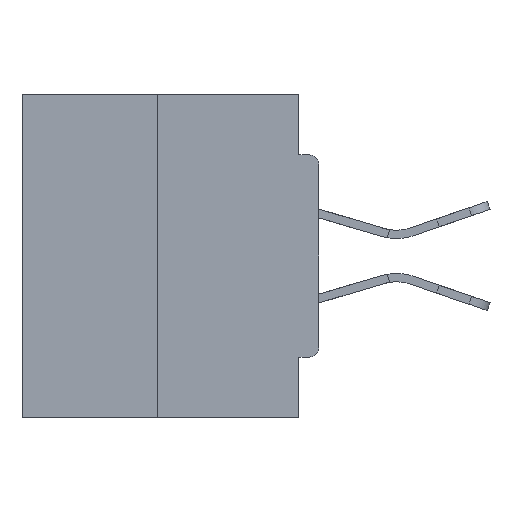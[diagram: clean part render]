
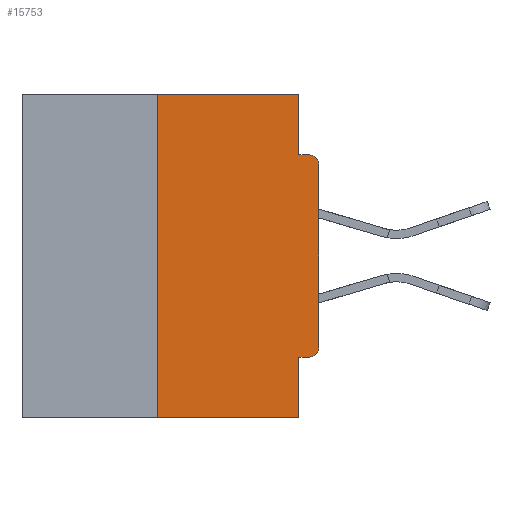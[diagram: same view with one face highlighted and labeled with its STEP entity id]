
A CAD part, left-side view. The second image highlights one B-rep face of the part: STEP entity #15753.
In plain terms, the highlighted planar face has unit normal (-1, 0, 0).
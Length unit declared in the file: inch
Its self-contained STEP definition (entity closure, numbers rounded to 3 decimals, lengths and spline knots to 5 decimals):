
#623 = VECTOR ( 'NONE', #2647, 39.37008 ) ;
#1178 = DIRECTION ( 'NONE',  ( 0., 0., -1. ) ) ;
#2207 = DIRECTION ( 'NONE',  ( 0., -1., 0. ) ) ;
#2476 = VERTEX_POINT ( 'NONE', #34500 ) ;
#2647 = DIRECTION ( 'NONE',  ( 0., 0., 1. ) ) ;
#2746 = VERTEX_POINT ( 'NONE', #12553 ) ;
#2925 = ORIENTED_EDGE ( 'NONE', *, *, #17171, .F. ) ;
#4962 = ORIENTED_EDGE ( 'NONE', *, *, #29750, .T. ) ;
#5063 = CARTESIAN_POINT ( 'NONE',  ( 0., 0., -0.3915 ) ) ;
#5082 = ORIENTED_EDGE ( 'NONE', *, *, #13976, .F. ) ;
#6606 = VERTEX_POINT ( 'NONE', #25374 ) ;
#6921 = VECTOR ( 'NONE', #8288, 39.37008 ) ;
#7028 = CARTESIAN_POINT ( 'NONE',  ( 0., 0.031, 0. ) ) ;
#7537 = ORIENTED_EDGE ( 'NONE', *, *, #27830, .T. ) ;
#7737 = LINE ( 'NONE', #21333, #19888 ) ;
#7827 = CARTESIAN_POINT ( 'NONE',  ( 0., 0., -0.4065 ) ) ;
#8288 = DIRECTION ( 'NONE',  ( 0., 0., -1. ) ) ;
#8445 = VECTOR ( 'NONE', #2207, 39.37008 ) ;
#8613 = DIRECTION ( 'NONE',  ( 0., 0., -1. ) ) ;
#9254 = VERTEX_POINT ( 'NONE', #29983 ) ;
#9478 = VERTEX_POINT ( 'NONE', #5063 ) ;
#9600 = LINE ( 'NONE', #31907, #33876 ) ;
#9910 = FACE_OUTER_BOUND ( 'NONE', #16501, .T. ) ;
#11803 = VECTOR ( 'NONE', #19693, 39.37008 ) ;
#11914 = DIRECTION ( 'NONE',  ( 0., -1., 0. ) ) ;
#12397 = DIRECTION ( 'NONE',  ( 0., 0., -1. ) ) ;
#12553 = CARTESIAN_POINT ( 'NONE',  ( 0., 0.031, -0.0935 ) ) ;
#13263 = LINE ( 'NONE', #17186, #31629 ) ;
#13328 = VERTEX_POINT ( 'NONE', #36318 ) ;
#13926 = AXIS2_PLACEMENT_3D ( 'NONE', #21272, #14971, #12397 ) ;
#13976 = EDGE_CURVE ( 'NONE', #31612, #2476, #16914, .T. ) ;
#14450 = EDGE_CURVE ( 'NONE', #9254, #31612, #35189, .T. ) ;
#14680 = LINE ( 'NONE', #28854, #6921 ) ;
#14771 = EDGE_CURVE ( 'NONE', #32378, #17305, #7737, .T. ) ;
#14971 = DIRECTION ( 'NONE',  ( -1., 0., 0. ) ) ;
#15753 = ADVANCED_FACE ( 'NONE', ( #9910 ), #24423, .F. ) ;
#15808 = CARTESIAN_POINT ( 'NONE',  ( 0., 0.46, 0. ) ) ;
#16501 = EDGE_LOOP ( 'NONE', ( #20566, #33619, #7537, #5082, #18240, #34674, #24476, #4962, #2925, #23330 ) ) ;
#16602 = LINE ( 'NONE', #35376, #623 ) ;
#16914 = LINE ( 'NONE', #29058, #33400 ) ;
#17171 = EDGE_CURVE ( 'NONE', #2746, #6606, #24956, .T. ) ;
#17186 = CARTESIAN_POINT ( 'NONE',  ( 0., 0.25, 0. ) ) ;
#17305 = VERTEX_POINT ( 'NONE', #7028 ) ;
#18240 = ORIENTED_EDGE ( 'NONE', *, *, #14450, .F. ) ;
#18448 = CARTESIAN_POINT ( 'NONE',  ( 0., 0.015, -0.1085 ) ) ;
#19629 = EDGE_CURVE ( 'NONE', #9478, #13328, #16602, .T. ) ;
#19693 = DIRECTION ( 'NONE',  ( 0., 1., 0. ) ) ;
#19888 = VECTOR ( 'NONE', #24511, 39.37008 ) ;
#20432 = DIRECTION ( 'NONE',  ( 0., 0., 1. ) ) ;
#20566 = ORIENTED_EDGE ( 'NONE', *, *, #14771, .F. ) ;
#21064 = DIRECTION ( 'NONE',  ( 0., 0., -1. ) ) ;
#21272 = CARTESIAN_POINT ( 'NONE',  ( 0., 0.015, -0.3915 ) ) ;
#21333 = CARTESIAN_POINT ( 'NONE',  ( 0., 0.46, 0. ) ) ;
#23330 = ORIENTED_EDGE ( 'NONE', *, *, #37208, .F. ) ;
#24423 = PLANE ( 'NONE',  #32478 ) ;
#24476 = ORIENTED_EDGE ( 'NONE', *, *, #19629, .T. ) ;
#24511 = DIRECTION ( 'NONE',  ( 0., -1., 0. ) ) ;
#24520 = CARTESIAN_POINT ( 'NONE',  ( 0., 0.25, -0.5 ) ) ;
#24956 = LINE ( 'NONE', #31365, #8445 ) ;
#25374 = CARTESIAN_POINT ( 'NONE',  ( 0., 0.015, -0.0935 ) ) ;
#27700 = CARTESIAN_POINT ( 'NONE',  ( 0., 0.031, -0.4065 ) ) ;
#27830 = EDGE_CURVE ( 'NONE', #30306, #2476, #9600, .T. ) ;
#27923 = EDGE_CURVE ( 'NONE', #9254, #9478, #37546, .T. ) ;
#28854 = CARTESIAN_POINT ( 'NONE',  ( 0., 0.031, 0. ) ) ;
#29058 = CARTESIAN_POINT ( 'NONE',  ( 0., 0.031, -0.5 ) ) ;
#29750 = EDGE_CURVE ( 'NONE', #13328, #6606, #31070, .T. ) ;
#29983 = CARTESIAN_POINT ( 'NONE',  ( 0., 0.015, -0.4065 ) ) ;
#30306 = VERTEX_POINT ( 'NONE', #24520 ) ;
#31070 = CIRCLE ( 'NONE', #35597, 0.015 ) ;
#31365 = CARTESIAN_POINT ( 'NONE',  ( 0., 0., -0.0935 ) ) ;
#31612 = VERTEX_POINT ( 'NONE', #27700 ) ;
#31629 = VECTOR ( 'NONE', #20432, 39.37008 ) ;
#31907 = CARTESIAN_POINT ( 'NONE',  ( 0., 0.46, -0.5 ) ) ;
#32378 = VERTEX_POINT ( 'NONE', #32543 ) ;
#32478 = AXIS2_PLACEMENT_3D ( 'NONE', #15808, #36313, #1178 ) ;
#32543 = CARTESIAN_POINT ( 'NONE',  ( 0., 0.25, 0. ) ) ;
#33400 = VECTOR ( 'NONE', #8613, 39.37008 ) ;
#33619 = ORIENTED_EDGE ( 'NONE', *, *, #37153, .F. ) ;
#33876 = VECTOR ( 'NONE', #11914, 39.37008 ) ;
#34500 = CARTESIAN_POINT ( 'NONE',  ( 0., 0.031, -0.5 ) ) ;
#34674 = ORIENTED_EDGE ( 'NONE', *, *, #27923, .T. ) ;
#35189 = LINE ( 'NONE', #7827, #11803 ) ;
#35376 = CARTESIAN_POINT ( 'NONE',  ( 0., 0., 0. ) ) ;
#35597 = AXIS2_PLACEMENT_3D ( 'NONE', #18448, #35638, #21064 ) ;
#35638 = DIRECTION ( 'NONE',  ( -1., 0., 0. ) ) ;
#36313 = DIRECTION ( 'NONE',  ( 1., 0., 0. ) ) ;
#36318 = CARTESIAN_POINT ( 'NONE',  ( 0., 0., -0.1085 ) ) ;
#37153 = EDGE_CURVE ( 'NONE', #30306, #32378, #13263, .T. ) ;
#37208 = EDGE_CURVE ( 'NONE', #17305, #2746, #14680, .T. ) ;
#37546 = CIRCLE ( 'NONE', #13926, 0.015 ) ;
